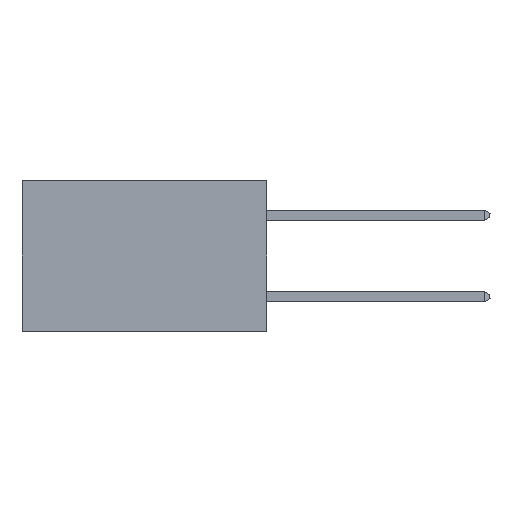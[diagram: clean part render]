
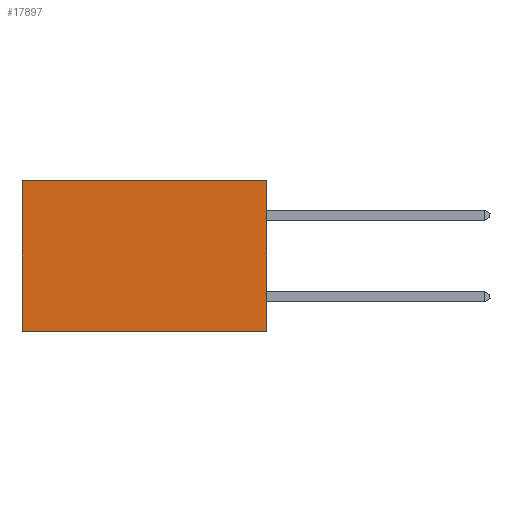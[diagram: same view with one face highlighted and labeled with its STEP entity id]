
A CAD part, left-side view. The second image highlights one B-rep face of the part: STEP entity #17897.
In plain terms, the highlighted planar face has unit normal (-1, 0, 0).
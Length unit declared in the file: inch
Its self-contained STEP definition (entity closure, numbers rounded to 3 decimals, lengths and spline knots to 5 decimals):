
#2066 = FACE_OUTER_BOUND ( 'NONE', #2629, .T. ) ;
#2175 = CARTESIAN_POINT ( 'NONE',  ( 0.2875, 0., 0. ) ) ;
#2629 = EDGE_LOOP ( 'NONE', ( #22649, #20777, #8383, #8413 ) ) ;
#3334 = CARTESIAN_POINT ( 'NONE',  ( 0.2875, 0.6, 0. ) ) ;
#4873 = PLANE ( 'NONE',  #6030 ) ;
#5335 = CARTESIAN_POINT ( 'NONE',  ( 0.2875, 0.6, 0. ) ) ;
#5726 = CARTESIAN_POINT ( 'NONE',  ( 0.2875, 0., -0.37 ) ) ;
#5745 = VERTEX_POINT ( 'NONE', #29704 ) ;
#6030 = AXIS2_PLACEMENT_3D ( 'NONE', #7216, #25703, #11843 ) ;
#6662 = VERTEX_POINT ( 'NONE', #8285 ) ;
#7216 = CARTESIAN_POINT ( 'NONE',  ( 0.2875, 0., 0. ) ) ;
#8207 = VERTEX_POINT ( 'NONE', #5335 ) ;
#8248 = CARTESIAN_POINT ( 'NONE',  ( 0.2875, 0., 0. ) ) ;
#8285 = CARTESIAN_POINT ( 'NONE',  ( 0.2875, 0., 0. ) ) ;
#8310 = VERTEX_POINT ( 'NONE', #5726 ) ;
#8383 = ORIENTED_EDGE ( 'NONE', *, *, #13798, .F. ) ;
#8413 = ORIENTED_EDGE ( 'NONE', *, *, #22720, .T. ) ;
#8453 = DIRECTION ( 'NONE',  ( 0., 0., -1. ) ) ;
#9233 = LINE ( 'NONE', #8248, #13196 ) ;
#11843 = DIRECTION ( 'NONE',  ( 0., 0., -1. ) ) ;
#13104 = LINE ( 'NONE', #3334, #25077 ) ;
#13196 = VECTOR ( 'NONE', #8453, 39.37008 ) ;
#13798 = EDGE_CURVE ( 'NONE', #6662, #8310, #9233, .T. ) ;
#13859 = VECTOR ( 'NONE', #25564, 39.37008 ) ;
#15102 = DIRECTION ( 'NONE',  ( 0., 0., -1. ) ) ;
#15474 = EDGE_CURVE ( 'NONE', #8207, #5745, #13104, .T. ) ;
#17897 = ADVANCED_FACE ( 'NONE', ( #2066 ), #4873, .F. ) ;
#18829 = CARTESIAN_POINT ( 'NONE',  ( 0.2875, 0., -0.37 ) ) ;
#19869 = LINE ( 'NONE', #2175, #28927 ) ;
#20777 = ORIENTED_EDGE ( 'NONE', *, *, #26147, .F. ) ;
#20784 = DIRECTION ( 'NONE',  ( 0., 1., 0. ) ) ;
#21119 = LINE ( 'NONE', #18829, #13859 ) ;
#22649 = ORIENTED_EDGE ( 'NONE', *, *, #15474, .T. ) ;
#22720 = EDGE_CURVE ( 'NONE', #6662, #8207, #19869, .T. ) ;
#25077 = VECTOR ( 'NONE', #15102, 39.37008 ) ;
#25564 = DIRECTION ( 'NONE',  ( 0., 1., 0. ) ) ;
#25703 = DIRECTION ( 'NONE',  ( 1., 0., 0. ) ) ;
#26147 = EDGE_CURVE ( 'NONE', #8310, #5745, #21119, .T. ) ;
#28927 = VECTOR ( 'NONE', #20784, 39.37008 ) ;
#29704 = CARTESIAN_POINT ( 'NONE',  ( 0.2875, 0.6, -0.37 ) ) ;
